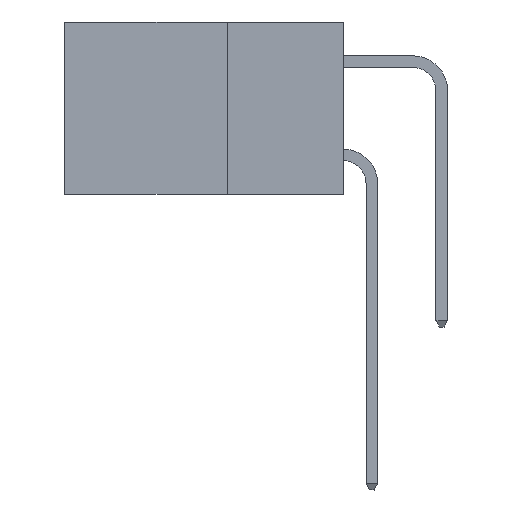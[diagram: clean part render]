
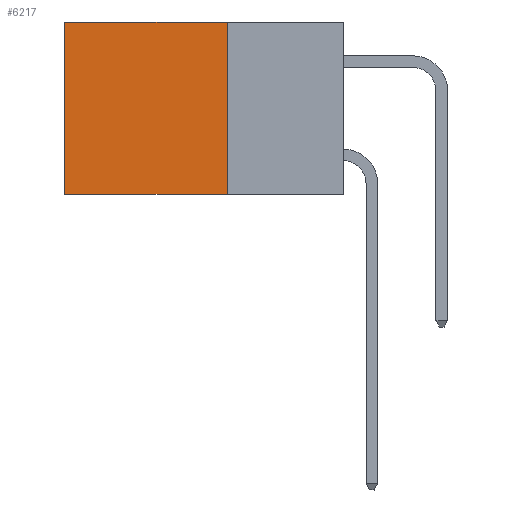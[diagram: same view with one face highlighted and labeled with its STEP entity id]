
A CAD part, left-side view. The second image highlights one B-rep face of the part: STEP entity #6217.
In plain terms, the highlighted planar face has unit normal (-1, 0, 0).
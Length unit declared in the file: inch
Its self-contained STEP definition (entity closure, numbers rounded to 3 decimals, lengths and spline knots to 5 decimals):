
#811 = DIRECTION ( 'NONE',  ( 0., 0., -1. ) ) ;
#1528 = VERTEX_POINT ( 'NONE', #17156 ) ;
#1604 = CARTESIAN_POINT ( 'NONE',  ( 0.298, 0.25, 0. ) ) ;
#2843 = CARTESIAN_POINT ( 'NONE',  ( 0.298, 0.25, 0. ) ) ;
#2908 = LINE ( 'NONE', #5535, #6275 ) ;
#3179 = CARTESIAN_POINT ( 'NONE',  ( 0.298, 0.25, 0. ) ) ;
#3616 = DIRECTION ( 'NONE',  ( 0., 1., 0. ) ) ;
#4255 = DIRECTION ( 'NONE',  ( 1., 0., 0. ) ) ;
#4772 = VECTOR ( 'NONE', #5296, 39.37008 ) ;
#5296 = DIRECTION ( 'NONE',  ( 0., 1., 0. ) ) ;
#5535 = CARTESIAN_POINT ( 'NONE',  ( 0.298, 0.25, -0.37 ) ) ;
#6123 = EDGE_CURVE ( 'NONE', #31771, #1528, #2908, .T. ) ;
#6217 = ADVANCED_FACE ( 'NONE', ( #20526 ), #11497, .F. ) ;
#6275 = VECTOR ( 'NONE', #3616, 39.37008 ) ;
#6529 = EDGE_LOOP ( 'NONE', ( #26215, #8618, #26666, #28101 ) ) ;
#6723 = DIRECTION ( 'NONE',  ( 0., 0., -1. ) ) ;
#8038 = VECTOR ( 'NONE', #20723, 39.37008 ) ;
#8618 = ORIENTED_EDGE ( 'NONE', *, *, #6123, .F. ) ;
#10840 = LINE ( 'NONE', #3179, #16241 ) ;
#11497 = PLANE ( 'NONE',  #26205 ) ;
#12620 = EDGE_CURVE ( 'NONE', #18703, #1528, #26829, .T. ) ;
#16061 = CARTESIAN_POINT ( 'NONE',  ( 0.298, 0.6, 0. ) ) ;
#16241 = VECTOR ( 'NONE', #811, 39.37008 ) ;
#17156 = CARTESIAN_POINT ( 'NONE',  ( 0.298, 0.6, -0.37 ) ) ;
#17735 = CARTESIAN_POINT ( 'NONE',  ( 0.298, 0.6, 0. ) ) ;
#18703 = VERTEX_POINT ( 'NONE', #17735 ) ;
#20526 = FACE_OUTER_BOUND ( 'NONE', #6529, .T. ) ;
#20723 = DIRECTION ( 'NONE',  ( 0., 0., -1. ) ) ;
#22667 = CARTESIAN_POINT ( 'NONE',  ( 0.298, 0.25, 0. ) ) ;
#23013 = VERTEX_POINT ( 'NONE', #22667 ) ;
#25432 = EDGE_CURVE ( 'NONE', #23013, #18703, #26254, .T. ) ;
#26205 = AXIS2_PLACEMENT_3D ( 'NONE', #1604, #4255, #6723 ) ;
#26215 = ORIENTED_EDGE ( 'NONE', *, *, #12620, .T. ) ;
#26254 = LINE ( 'NONE', #2843, #4772 ) ;
#26666 = ORIENTED_EDGE ( 'NONE', *, *, #26807, .F. ) ;
#26807 = EDGE_CURVE ( 'NONE', #23013, #31771, #10840, .T. ) ;
#26829 = LINE ( 'NONE', #16061, #8038 ) ;
#28101 = ORIENTED_EDGE ( 'NONE', *, *, #25432, .T. ) ;
#30246 = CARTESIAN_POINT ( 'NONE',  ( 0.298, 0.25, -0.37 ) ) ;
#31771 = VERTEX_POINT ( 'NONE', #30246 ) ;
